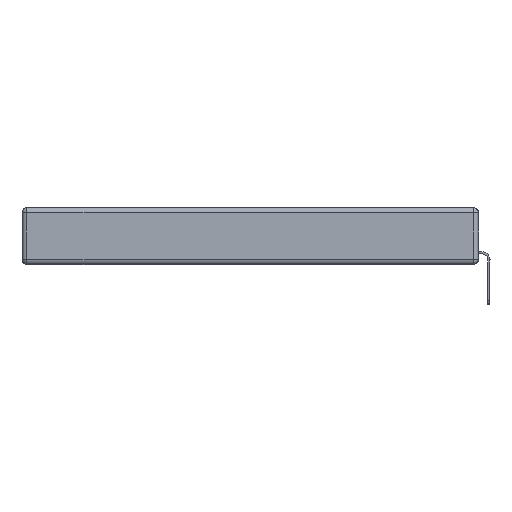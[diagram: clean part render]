
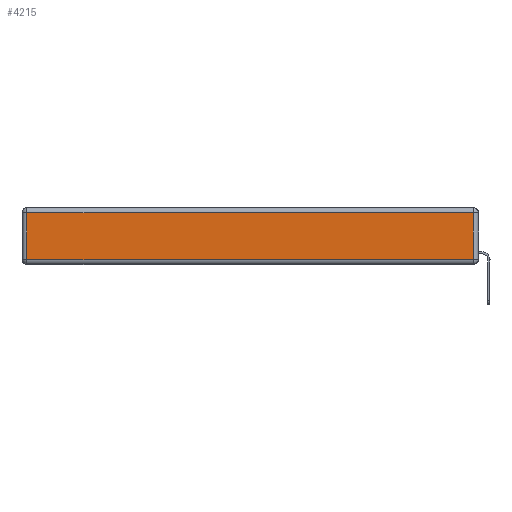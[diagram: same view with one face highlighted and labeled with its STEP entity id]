
A CAD part, left-side view. The second image highlights one B-rep face of the part: STEP entity #4215.
In plain terms, the highlighted planar face has unit normal (-1, 0, 0).
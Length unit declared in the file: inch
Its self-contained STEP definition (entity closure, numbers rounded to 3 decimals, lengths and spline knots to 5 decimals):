
#44 = EDGE_CURVE ( 'NONE', #22966, #18362, #18488, .T. ) ;
#274 = DIRECTION ( 'NONE',  ( 0., 0., 1. ) ) ;
#1150 = CARTESIAN_POINT ( 'NONE',  ( 0., 0.03, -0.313 ) ) ;
#1796 = DIRECTION ( 'NONE',  ( 0., -1., 0. ) ) ;
#2179 = EDGE_CURVE ( 'NONE', #16361, #22966, #13273, .T. ) ;
#2223 = EDGE_LOOP ( 'NONE', ( #21828, #9686, #7733, #20343 ) ) ;
#3190 = CARTESIAN_POINT ( 'NONE',  ( 0., 2.72, -0.343 ) ) ;
#3651 = CARTESIAN_POINT ( 'NONE',  ( 0., 0., -0.343 ) ) ;
#3897 = DIRECTION ( 'NONE',  ( -1., 0., 0. ) ) ;
#4160 = VECTOR ( 'NONE', #1796, 39.37008 ) ;
#4191 = CARTESIAN_POINT ( 'NONE',  ( 0., 0.03, -0.343 ) ) ;
#4215 = ADVANCED_FACE ( 'NONE', ( #17481 ), #11579, .T. ) ;
#4631 = VECTOR ( 'NONE', #274, 39.37008 ) ;
#5268 = EDGE_CURVE ( 'NONE', #5677, #16361, #13627, .T. ) ;
#5290 = AXIS2_PLACEMENT_3D ( 'NONE', #3651, #3897, #19301 ) ;
#5677 = VERTEX_POINT ( 'NONE', #12354 ) ;
#7733 = ORIENTED_EDGE ( 'NONE', *, *, #44, .T. ) ;
#7818 = VECTOR ( 'NONE', #8423, 39.37008 ) ;
#8423 = DIRECTION ( 'NONE',  ( 0., 1., 0. ) ) ;
#9686 = ORIENTED_EDGE ( 'NONE', *, *, #2179, .T. ) ;
#11579 = PLANE ( 'NONE',  #5290 ) ;
#12354 = CARTESIAN_POINT ( 'NONE',  ( 0., 2.72, -0.313 ) ) ;
#13273 = LINE ( 'NONE', #4191, #4631 ) ;
#13626 = VECTOR ( 'NONE', #18423, 39.37008 ) ;
#13627 = LINE ( 'NONE', #15497, #4160 ) ;
#15497 = CARTESIAN_POINT ( 'NONE',  ( 0., 0., -0.313 ) ) ;
#16361 = VERTEX_POINT ( 'NONE', #1150 ) ;
#17032 = CARTESIAN_POINT ( 'NONE',  ( 0., 2.72, -0.03 ) ) ;
#17481 = FACE_OUTER_BOUND ( 'NONE', #2223, .T. ) ;
#18355 = CARTESIAN_POINT ( 'NONE',  ( 0., 2.75, -0.03 ) ) ;
#18362 = VERTEX_POINT ( 'NONE', #17032 ) ;
#18423 = DIRECTION ( 'NONE',  ( 0., 0., -1. ) ) ;
#18488 = LINE ( 'NONE', #18355, #7818 ) ;
#18701 = CARTESIAN_POINT ( 'NONE',  ( 0., 0.03, -0.03 ) ) ;
#19301 = DIRECTION ( 'NONE',  ( 0., 0., 1. ) ) ;
#20343 = ORIENTED_EDGE ( 'NONE', *, *, #24598, .T. ) ;
#21828 = ORIENTED_EDGE ( 'NONE', *, *, #5268, .T. ) ;
#22966 = VERTEX_POINT ( 'NONE', #18701 ) ;
#24598 = EDGE_CURVE ( 'NONE', #18362, #5677, #24754, .T. ) ;
#24754 = LINE ( 'NONE', #3190, #13626 ) ;
